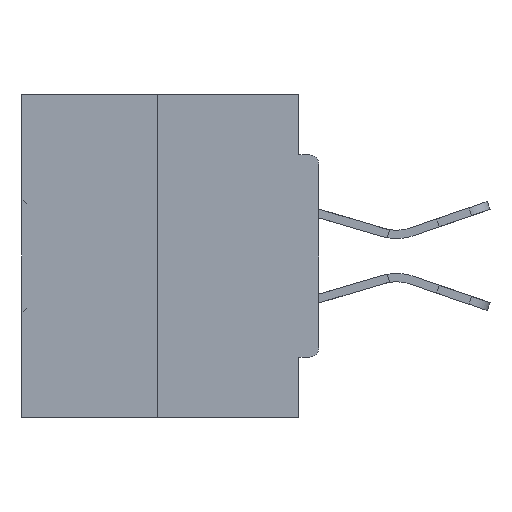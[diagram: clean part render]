
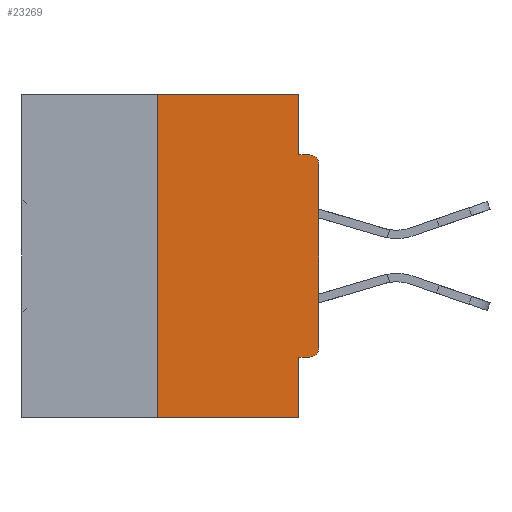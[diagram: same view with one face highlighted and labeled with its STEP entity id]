
A CAD part, left-side view. The second image highlights one B-rep face of the part: STEP entity #23269.
In plain terms, the highlighted planar face has unit normal (-1, 0, 0).
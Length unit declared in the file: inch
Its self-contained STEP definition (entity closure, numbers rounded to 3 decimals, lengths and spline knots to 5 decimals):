
#190 = CARTESIAN_POINT ( 'NONE',  ( 0., 0.015, -0.3915 ) ) ;
#604 = ORIENTED_EDGE ( 'NONE', *, *, #17495, .F. ) ;
#1095 = VERTEX_POINT ( 'NONE', #40561 ) ;
#1455 = ORIENTED_EDGE ( 'NONE', *, *, #17420, .F. ) ;
#1559 = VERTEX_POINT ( 'NONE', #19537 ) ;
#1670 = AXIS2_PLACEMENT_3D ( 'NONE', #190, #4382, #39193 ) ;
#1732 = VERTEX_POINT ( 'NONE', #27803 ) ;
#2858 = EDGE_CURVE ( 'NONE', #7215, #33088, #5651, .T. ) ;
#3976 = CARTESIAN_POINT ( 'NONE',  ( 0., 0., 0. ) ) ;
#4280 = EDGE_CURVE ( 'NONE', #32467, #11203, #38336, .T. ) ;
#4382 = DIRECTION ( 'NONE',  ( -1., 0., 0. ) ) ;
#4601 = LINE ( 'NONE', #23570, #31306 ) ;
#5113 = VECTOR ( 'NONE', #5843, 39.37008 ) ;
#5533 = EDGE_CURVE ( 'NONE', #7215, #1732, #18748, .T. ) ;
#5651 = LINE ( 'NONE', #27134, #5113 ) ;
#5843 = DIRECTION ( 'NONE',  ( 0., 1., 0. ) ) ;
#5956 = ORIENTED_EDGE ( 'NONE', *, *, #36483, .T. ) ;
#7215 = VERTEX_POINT ( 'NONE', #14404 ) ;
#7251 = ORIENTED_EDGE ( 'NONE', *, *, #5533, .T. ) ;
#7726 = DIRECTION ( 'NONE',  ( 0., 0., -1. ) ) ;
#9341 = VECTOR ( 'NONE', #38030, 39.37008 ) ;
#9709 = VERTEX_POINT ( 'NONE', #11276 ) ;
#10324 = CARTESIAN_POINT ( 'NONE',  ( 0., 0.46, 0. ) ) ;
#11203 = VERTEX_POINT ( 'NONE', #23147 ) ;
#11276 = CARTESIAN_POINT ( 'NONE',  ( 0., 0., -0.1085 ) ) ;
#11736 = ORIENTED_EDGE ( 'NONE', *, *, #34863, .F. ) ;
#12602 = VECTOR ( 'NONE', #13917, 39.37008 ) ;
#13809 = CARTESIAN_POINT ( 'NONE',  ( 0., 0.25, -0.5 ) ) ;
#13917 = DIRECTION ( 'NONE',  ( 0., 0., -1. ) ) ;
#14404 = CARTESIAN_POINT ( 'NONE',  ( 0., 0.015, -0.4065 ) ) ;
#15179 = AXIS2_PLACEMENT_3D ( 'NONE', #43178, #32504, #7726 ) ;
#15451 = ORIENTED_EDGE ( 'NONE', *, *, #2858, .F. ) ;
#15626 = DIRECTION ( 'NONE',  ( 0., -1., 0. ) ) ;
#16765 = ORIENTED_EDGE ( 'NONE', *, *, #37604, .T. ) ;
#16897 = CARTESIAN_POINT ( 'NONE',  ( 0., 0.031, 0. ) ) ;
#16983 = DIRECTION ( 'NONE',  ( 0., 0., -1. ) ) ;
#17420 = EDGE_CURVE ( 'NONE', #32467, #35096, #18689, .T. ) ;
#17495 = EDGE_CURVE ( 'NONE', #33088, #11203, #22055, .T. ) ;
#18689 = LINE ( 'NONE', #30540, #34914 ) ;
#18748 = CIRCLE ( 'NONE', #1670, 0.015 ) ;
#19235 = DIRECTION ( 'NONE',  ( 0., 0., -1. ) ) ;
#19334 = ORIENTED_EDGE ( 'NONE', *, *, #35606, .F. ) ;
#19537 = CARTESIAN_POINT ( 'NONE',  ( 0., 0.031, -0.0935 ) ) ;
#19752 = CIRCLE ( 'NONE', #15179, 0.015 ) ;
#19761 = ORIENTED_EDGE ( 'NONE', *, *, #39202, .F. ) ;
#22055 = LINE ( 'NONE', #24851, #12602 ) ;
#23014 = DIRECTION ( 'NONE',  ( 0., 0., 1. ) ) ;
#23147 = CARTESIAN_POINT ( 'NONE',  ( 0., 0.031, -0.5 ) ) ;
#23269 = ADVANCED_FACE ( 'NONE', ( #24803 ), #39623, .F. ) ;
#23570 = CARTESIAN_POINT ( 'NONE',  ( 0., 0.031, 0. ) ) ;
#24803 = FACE_OUTER_BOUND ( 'NONE', #41648, .T. ) ;
#24851 = CARTESIAN_POINT ( 'NONE',  ( 0., 0.031, -0.5 ) ) ;
#24951 = DIRECTION ( 'NONE',  ( 0., 0., 1. ) ) ;
#26704 = CARTESIAN_POINT ( 'NONE',  ( 0., 0.031, -0.4065 ) ) ;
#26906 = LINE ( 'NONE', #3976, #35257 ) ;
#27134 = CARTESIAN_POINT ( 'NONE',  ( 0., 0., -0.4065 ) ) ;
#27803 = CARTESIAN_POINT ( 'NONE',  ( 0., 0., -0.3915 ) ) ;
#28762 = ORIENTED_EDGE ( 'NONE', *, *, #4280, .T. ) ;
#28797 = CARTESIAN_POINT ( 'NONE',  ( 0., 0.25, 0. ) ) ;
#28863 = VECTOR ( 'NONE', #15626, 39.37008 ) ;
#30448 = VECTOR ( 'NONE', #35242, 39.37008 ) ;
#30540 = CARTESIAN_POINT ( 'NONE',  ( 0., 0.25, 0. ) ) ;
#31041 = CARTESIAN_POINT ( 'NONE',  ( 0., 0., -0.0935 ) ) ;
#31306 = VECTOR ( 'NONE', #16983, 39.37008 ) ;
#31402 = AXIS2_PLACEMENT_3D ( 'NONE', #34718, #35304, #19235 ) ;
#32467 = VERTEX_POINT ( 'NONE', #13809 ) ;
#32504 = DIRECTION ( 'NONE',  ( -1., 0., 0. ) ) ;
#33088 = VERTEX_POINT ( 'NONE', #26704 ) ;
#34718 = CARTESIAN_POINT ( 'NONE',  ( 0., 0.46, 0. ) ) ;
#34863 = EDGE_CURVE ( 'NONE', #1559, #1095, #37716, .T. ) ;
#34914 = VECTOR ( 'NONE', #23014, 39.37008 ) ;
#35096 = VERTEX_POINT ( 'NONE', #28797 ) ;
#35242 = DIRECTION ( 'NONE',  ( 0., -1., 0. ) ) ;
#35257 = VECTOR ( 'NONE', #24951, 39.37008 ) ;
#35304 = DIRECTION ( 'NONE',  ( 1., 0., 0. ) ) ;
#35459 = VERTEX_POINT ( 'NONE', #16897 ) ;
#35606 = EDGE_CURVE ( 'NONE', #35096, #35459, #42667, .T. ) ;
#36483 = EDGE_CURVE ( 'NONE', #9709, #1095, #19752, .T. ) ;
#37319 = CARTESIAN_POINT ( 'NONE',  ( 0., 0.46, -0.5 ) ) ;
#37604 = EDGE_CURVE ( 'NONE', #1732, #9709, #26906, .T. ) ;
#37716 = LINE ( 'NONE', #31041, #9341 ) ;
#38030 = DIRECTION ( 'NONE',  ( 0., -1., 0. ) ) ;
#38336 = LINE ( 'NONE', #37319, #28863 ) ;
#39193 = DIRECTION ( 'NONE',  ( 0., 0., -1. ) ) ;
#39202 = EDGE_CURVE ( 'NONE', #35459, #1559, #4601, .T. ) ;
#39623 = PLANE ( 'NONE',  #31402 ) ;
#40561 = CARTESIAN_POINT ( 'NONE',  ( 0., 0.015, -0.0935 ) ) ;
#41648 = EDGE_LOOP ( 'NONE', ( #19334, #1455, #28762, #604, #15451, #7251, #16765, #5956, #11736, #19761 ) ) ;
#42667 = LINE ( 'NONE', #10324, #30448 ) ;
#43178 = CARTESIAN_POINT ( 'NONE',  ( 0., 0.015, -0.1085 ) ) ;
